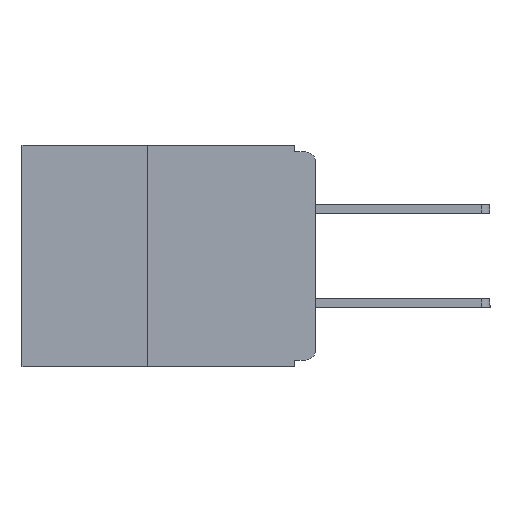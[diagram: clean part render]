
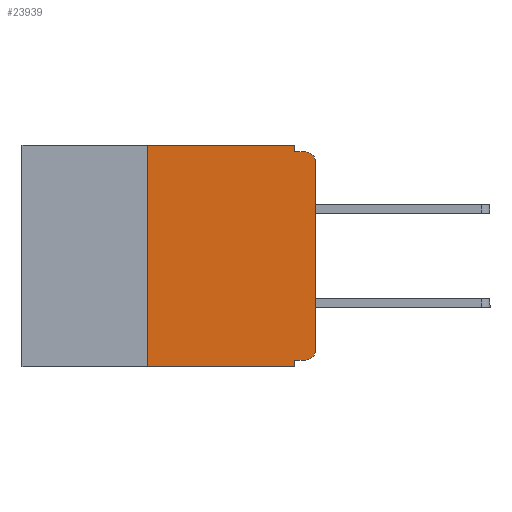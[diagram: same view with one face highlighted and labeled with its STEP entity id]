
A CAD part, left-side view. The second image highlights one B-rep face of the part: STEP entity #23939.
In plain terms, the highlighted planar face has unit normal (-1, 0, 0).
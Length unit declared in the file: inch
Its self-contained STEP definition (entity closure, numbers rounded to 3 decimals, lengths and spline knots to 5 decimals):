
#367 = EDGE_CURVE ( 'NONE', #26374, #10697, #4256, .T. ) ;
#617 = DIRECTION ( 'NONE',  ( 0., 0., -1. ) ) ;
#803 = ORIENTED_EDGE ( 'NONE', *, *, #7773, .F. ) ;
#818 = ORIENTED_EDGE ( 'NONE', *, *, #31160, .F. ) ;
#829 = CARTESIAN_POINT ( 'NONE',  ( 0., 0.25, -0.33 ) ) ;
#2006 = CARTESIAN_POINT ( 'NONE',  ( 0., 0.031, -0.01 ) ) ;
#2117 = VECTOR ( 'NONE', #25588, 39.37008 ) ;
#2251 = VECTOR ( 'NONE', #31579, 39.37008 ) ;
#2364 = LINE ( 'NONE', #20823, #30071 ) ;
#2657 = DIRECTION ( 'NONE',  ( -1., 0., 0. ) ) ;
#2755 = VERTEX_POINT ( 'NONE', #6490 ) ;
#2853 = CARTESIAN_POINT ( 'NONE',  ( 0., 0., -0.32 ) ) ;
#3141 = FACE_OUTER_BOUND ( 'NONE', #6214, .T. ) ;
#3918 = AXIS2_PLACEMENT_3D ( 'NONE', #28160, #28126, #27729 ) ;
#4256 = CIRCLE ( 'NONE', #3918, 0.015 ) ;
#4948 = CARTESIAN_POINT ( 'NONE',  ( 0., 0., 0. ) ) ;
#5475 = VERTEX_POINT ( 'NONE', #829 ) ;
#5545 = DIRECTION ( 'NONE',  ( 0., 1., 0. ) ) ;
#5587 = DIRECTION ( 'NONE',  ( 0., 0., 1. ) ) ;
#6214 = EDGE_LOOP ( 'NONE', ( #18173, #14783, #803, #19185, #25565, #22888, #32152, #33214, #818, #19652 ) ) ;
#6490 = CARTESIAN_POINT ( 'NONE',  ( 0., 0.25, 0. ) ) ;
#6652 = LINE ( 'NONE', #4948, #13629 ) ;
#6798 = AXIS2_PLACEMENT_3D ( 'NONE', #28765, #13244, #31269 ) ;
#7668 = CARTESIAN_POINT ( 'NONE',  ( 0., 0., -0.025 ) ) ;
#7773 = EDGE_CURVE ( 'NONE', #10080, #12317, #2364, .T. ) ;
#7952 = VERTEX_POINT ( 'NONE', #7668 ) ;
#9445 = CARTESIAN_POINT ( 'NONE',  ( 0., 0.031, 0. ) ) ;
#9616 = CARTESIAN_POINT ( 'NONE',  ( 0., 0.031, 0. ) ) ;
#9908 = VERTEX_POINT ( 'NONE', #9445 ) ;
#9995 = LINE ( 'NONE', #12613, #2117 ) ;
#9997 = EDGE_CURVE ( 'NONE', #10697, #7952, #6652, .T. ) ;
#10080 = VERTEX_POINT ( 'NONE', #2006 ) ;
#10489 = EDGE_CURVE ( 'NONE', #5475, #12829, #18969, .T. ) ;
#10697 = VERTEX_POINT ( 'NONE', #16922 ) ;
#11484 = EDGE_CURVE ( 'NONE', #9908, #10080, #27735, .T. ) ;
#11950 = VECTOR ( 'NONE', #26422, 39.37008 ) ;
#12317 = VERTEX_POINT ( 'NONE', #18670 ) ;
#12613 = CARTESIAN_POINT ( 'NONE',  ( 0., 0.437, 0. ) ) ;
#12829 = VERTEX_POINT ( 'NONE', #23391 ) ;
#13244 = DIRECTION ( 'NONE',  ( 1., 0., 0. ) ) ;
#13629 = VECTOR ( 'NONE', #5587, 39.37008 ) ;
#14783 = ORIENTED_EDGE ( 'NONE', *, *, #26816, .T. ) ;
#14917 = EDGE_CURVE ( 'NONE', #2755, #9908, #9995, .T. ) ;
#16006 = CARTESIAN_POINT ( 'NONE',  ( 0., 0.437, -0.33 ) ) ;
#16922 = CARTESIAN_POINT ( 'NONE',  ( 0., 0., -0.305 ) ) ;
#17452 = DIRECTION ( 'NONE',  ( 0., 0., -1. ) ) ;
#17953 = VECTOR ( 'NONE', #5545, 39.37008 ) ;
#18173 = ORIENTED_EDGE ( 'NONE', *, *, #9997, .T. ) ;
#18466 = CARTESIAN_POINT ( 'NONE',  ( 0., 0.015, -0.025 ) ) ;
#18572 = CARTESIAN_POINT ( 'NONE',  ( 0., 0.031, -0.32 ) ) ;
#18670 = CARTESIAN_POINT ( 'NONE',  ( 0., 0.015, -0.01 ) ) ;
#18969 = LINE ( 'NONE', #16006, #11950 ) ;
#19185 = ORIENTED_EDGE ( 'NONE', *, *, #11484, .F. ) ;
#19652 = ORIENTED_EDGE ( 'NONE', *, *, #367, .T. ) ;
#20823 = CARTESIAN_POINT ( 'NONE',  ( 0., 0., -0.01 ) ) ;
#20955 = VECTOR ( 'NONE', #17452, 39.37008 ) ;
#21091 = DIRECTION ( 'NONE',  ( 0., 0., -1. ) ) ;
#22379 = DIRECTION ( 'NONE',  ( 0., -1., 0. ) ) ;
#22888 = ORIENTED_EDGE ( 'NONE', *, *, #31206, .F. ) ;
#23235 = LINE ( 'NONE', #26520, #2251 ) ;
#23391 = CARTESIAN_POINT ( 'NONE',  ( 0., 0.031, -0.33 ) ) ;
#23902 = CIRCLE ( 'NONE', #27785, 0.015 ) ;
#23939 = ADVANCED_FACE ( 'NONE', ( #3141 ), #26196, .F. ) ;
#24458 = CARTESIAN_POINT ( 'NONE',  ( 0., 0.015, -0.32 ) ) ;
#25565 = ORIENTED_EDGE ( 'NONE', *, *, #14917, .F. ) ;
#25588 = DIRECTION ( 'NONE',  ( 0., -1., 0. ) ) ;
#26196 = PLANE ( 'NONE',  #6798 ) ;
#26374 = VERTEX_POINT ( 'NONE', #24458 ) ;
#26422 = DIRECTION ( 'NONE',  ( 0., -1., 0. ) ) ;
#26429 = LINE ( 'NONE', #2853, #17953 ) ;
#26520 = CARTESIAN_POINT ( 'NONE',  ( 0., 0.25, -0.33 ) ) ;
#26816 = EDGE_CURVE ( 'NONE', #7952, #12317, #23902, .T. ) ;
#27729 = DIRECTION ( 'NONE',  ( 0., 0., -1. ) ) ;
#27735 = LINE ( 'NONE', #9616, #20955 ) ;
#27785 = AXIS2_PLACEMENT_3D ( 'NONE', #18466, #2657, #21091 ) ;
#27878 = EDGE_CURVE ( 'NONE', #32357, #12829, #32503, .T. ) ;
#28126 = DIRECTION ( 'NONE',  ( -1., 0., 0. ) ) ;
#28160 = CARTESIAN_POINT ( 'NONE',  ( 0., 0.015, -0.305 ) ) ;
#28765 = CARTESIAN_POINT ( 'NONE',  ( 0., 0.437, 0. ) ) ;
#30071 = VECTOR ( 'NONE', #22379, 39.37008 ) ;
#30178 = VECTOR ( 'NONE', #617, 39.37008 ) ;
#31160 = EDGE_CURVE ( 'NONE', #26374, #32357, #26429, .T. ) ;
#31206 = EDGE_CURVE ( 'NONE', #5475, #2755, #23235, .T. ) ;
#31269 = DIRECTION ( 'NONE',  ( 0., 0., -1. ) ) ;
#31579 = DIRECTION ( 'NONE',  ( 0., 0., 1. ) ) ;
#31807 = CARTESIAN_POINT ( 'NONE',  ( 0., 0.031, -0.33 ) ) ;
#32152 = ORIENTED_EDGE ( 'NONE', *, *, #10489, .T. ) ;
#32357 = VERTEX_POINT ( 'NONE', #18572 ) ;
#32503 = LINE ( 'NONE', #31807, #30178 ) ;
#33214 = ORIENTED_EDGE ( 'NONE', *, *, #27878, .F. ) ;
